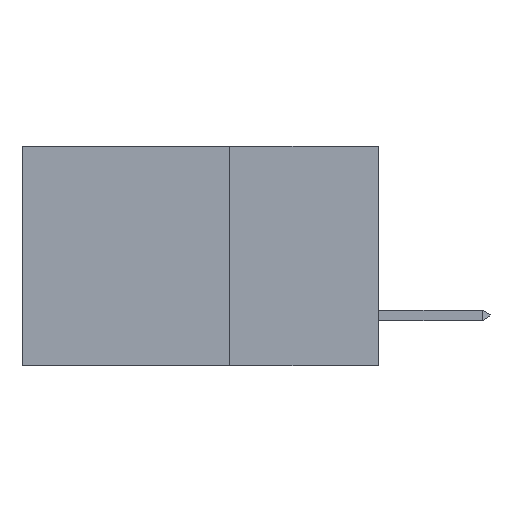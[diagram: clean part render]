
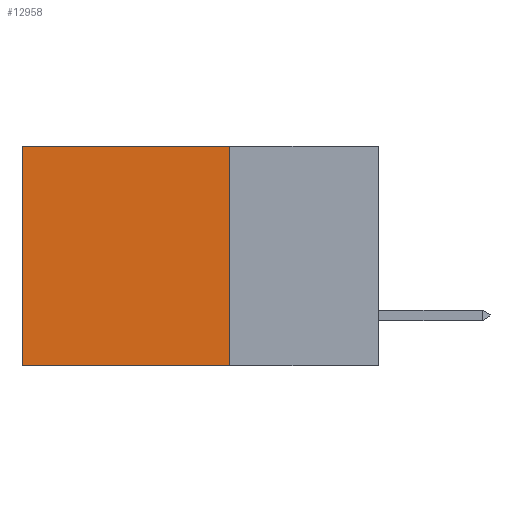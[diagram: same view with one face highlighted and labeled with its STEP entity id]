
A CAD part, left-side view. The second image highlights one B-rep face of the part: STEP entity #12958.
In plain terms, the highlighted planar face has unit normal (-1, 0, 0).
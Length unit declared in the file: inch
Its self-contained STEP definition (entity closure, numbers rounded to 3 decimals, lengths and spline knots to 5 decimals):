
#2205 = EDGE_CURVE ( 'NONE', #15796, #18111, #17818, .T. ) ;
#5149 = CARTESIAN_POINT ( 'NONE',  ( 0.2615, 0.6, 0. ) ) ;
#5736 = LINE ( 'NONE', #13921, #19020 ) ;
#6297 = DIRECTION ( 'NONE',  ( 0., 1., 0. ) ) ;
#6426 = LINE ( 'NONE', #14365, #8085 ) ;
#6973 = CARTESIAN_POINT ( 'NONE',  ( 0.2615, 0.25, 0. ) ) ;
#7907 = DIRECTION ( 'NONE',  ( 0., 0., -1. ) ) ;
#8085 = VECTOR ( 'NONE', #6297, 39.37008 ) ;
#8319 = ORIENTED_EDGE ( 'NONE', *, *, #2205, .F. ) ;
#8699 = ORIENTED_EDGE ( 'NONE', *, *, #10858, .T. ) ;
#9060 = FACE_OUTER_BOUND ( 'NONE', #15513, .T. ) ;
#9185 = DIRECTION ( 'NONE',  ( 1., 0., 0. ) ) ;
#9670 = VERTEX_POINT ( 'NONE', #5149 ) ;
#9875 = AXIS2_PLACEMENT_3D ( 'NONE', #22921, #9185, #11090 ) ;
#10858 = EDGE_CURVE ( 'NONE', #9670, #18111, #5736, .T. ) ;
#11090 = DIRECTION ( 'NONE',  ( 0., 0., -1. ) ) ;
#12435 = CARTESIAN_POINT ( 'NONE',  ( 0.2615, 0.25, -0.37 ) ) ;
#12538 = CARTESIAN_POINT ( 'NONE',  ( 0.2615, 0.25, -0.37 ) ) ;
#12958 = ADVANCED_FACE ( 'NONE', ( #9060 ), #15468, .F. ) ;
#13909 = ORIENTED_EDGE ( 'NONE', *, *, #21492, .T. ) ;
#13921 = CARTESIAN_POINT ( 'NONE',  ( 0.2615, 0.6, -0.37 ) ) ;
#14365 = CARTESIAN_POINT ( 'NONE',  ( 0.2615, 0.25, 0. ) ) ;
#14618 = VECTOR ( 'NONE', #21665, 39.37008 ) ;
#15468 = PLANE ( 'NONE',  #9875 ) ;
#15513 = EDGE_LOOP ( 'NONE', ( #8699, #8319, #24475, #13909 ) ) ;
#15796 = VERTEX_POINT ( 'NONE', #12538 ) ;
#17818 = LINE ( 'NONE', #17950, #14618 ) ;
#17950 = CARTESIAN_POINT ( 'NONE',  ( 0.2615, 0.25, -0.37 ) ) ;
#18111 = VERTEX_POINT ( 'NONE', #23430 ) ;
#18361 = DIRECTION ( 'NONE',  ( 0., 0., -1. ) ) ;
#19020 = VECTOR ( 'NONE', #7907, 39.37008 ) ;
#20415 = LINE ( 'NONE', #12435, #21198 ) ;
#21198 = VECTOR ( 'NONE', #18361, 39.37008 ) ;
#21378 = EDGE_CURVE ( 'NONE', #22300, #15796, #20415, .T. ) ;
#21492 = EDGE_CURVE ( 'NONE', #22300, #9670, #6426, .T. ) ;
#21665 = DIRECTION ( 'NONE',  ( 0., 1., 0. ) ) ;
#22300 = VERTEX_POINT ( 'NONE', #6973 ) ;
#22921 = CARTESIAN_POINT ( 'NONE',  ( 0.2615, 0.25, -0.37 ) ) ;
#23430 = CARTESIAN_POINT ( 'NONE',  ( 0.2615, 0.6, -0.37 ) ) ;
#24475 = ORIENTED_EDGE ( 'NONE', *, *, #21378, .F. ) ;
